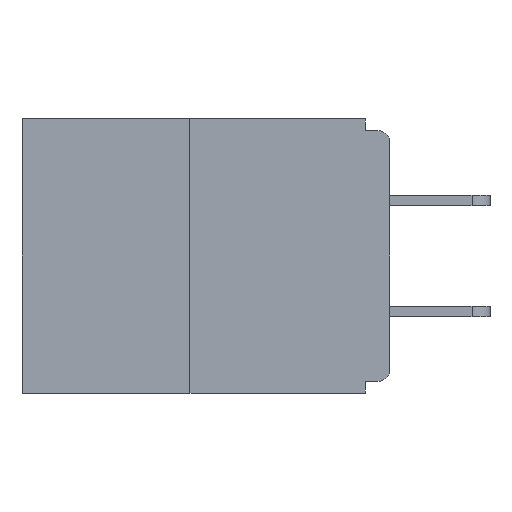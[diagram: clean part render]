
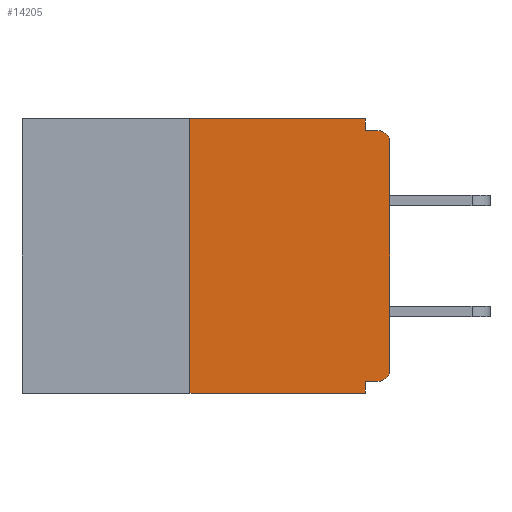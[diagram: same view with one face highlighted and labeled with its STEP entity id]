
A CAD part, left-side view. The second image highlights one B-rep face of the part: STEP entity #14205.
In plain terms, the highlighted planar face has unit normal (-1, 0, 0).
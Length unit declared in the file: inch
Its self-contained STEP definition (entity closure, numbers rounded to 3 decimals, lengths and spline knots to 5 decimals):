
#158 = CARTESIAN_POINT ( 'NONE',  ( 0., 0.015, -0.328 ) ) ;
#215 = CARTESIAN_POINT ( 'NONE',  ( 0., 0.25, 0. ) ) ;
#229 = EDGE_CURVE ( 'NONE', #11083, #8992, #6407, .T. ) ;
#235 = CARTESIAN_POINT ( 'NONE',  ( 0., 0.46, 0. ) ) ;
#699 = VECTOR ( 'NONE', #16931, 39.37008 ) ;
#839 = AXIS2_PLACEMENT_3D ( 'NONE', #7268, #9706, #13663 ) ;
#892 = VECTOR ( 'NONE', #11064, 39.37008 ) ;
#1254 = AXIS2_PLACEMENT_3D ( 'NONE', #10747, #15986, #8151 ) ;
#1256 = EDGE_CURVE ( 'NONE', #16691, #2936, #14068, .T. ) ;
#1741 = LINE ( 'NONE', #15733, #16290 ) ;
#1963 = DIRECTION ( 'NONE',  ( 0., -1., 0. ) ) ;
#2373 = AXIS2_PLACEMENT_3D ( 'NONE', #235, #15900, #2835 ) ;
#2428 = ORIENTED_EDGE ( 'NONE', *, *, #229, .F. ) ;
#2693 = LINE ( 'NONE', #5955, #9291 ) ;
#2835 = DIRECTION ( 'NONE',  ( 0., 0., -1. ) ) ;
#2936 = VERTEX_POINT ( 'NONE', #3466 ) ;
#3057 = EDGE_CURVE ( 'NONE', #14549, #4964, #15224, .T. ) ;
#3086 = LINE ( 'NONE', #5549, #16845 ) ;
#3451 = CARTESIAN_POINT ( 'NONE',  ( 0., 0.25, 0. ) ) ;
#3466 = CARTESIAN_POINT ( 'NONE',  ( 0., 0., -0.03 ) ) ;
#3746 = EDGE_CURVE ( 'NONE', #7110, #16691, #11566, .T. ) ;
#3866 = DIRECTION ( 'NONE',  ( 0., 0., -1. ) ) ;
#4085 = CARTESIAN_POINT ( 'NONE',  ( 0., 0.25, -0.343 ) ) ;
#4459 = CARTESIAN_POINT ( 'NONE',  ( 0., 0.031, -0.328 ) ) ;
#4520 = VECTOR ( 'NONE', #1963, 39.37008 ) ;
#4844 = EDGE_CURVE ( 'NONE', #7110, #6276, #3086, .T. ) ;
#4888 = DIRECTION ( 'NONE',  ( 0., -1., 0. ) ) ;
#4964 = VERTEX_POINT ( 'NONE', #3451 ) ;
#5214 = DIRECTION ( 'NONE',  ( 0., 0., 1. ) ) ;
#5549 = CARTESIAN_POINT ( 'NONE',  ( 0., 0., -0.328 ) ) ;
#5955 = CARTESIAN_POINT ( 'NONE',  ( 0., 0.46, 0. ) ) ;
#6276 = VERTEX_POINT ( 'NONE', #4459 ) ;
#6407 = LINE ( 'NONE', #13141, #699 ) ;
#6719 = PLANE ( 'NONE',  #2373 ) ;
#6796 = ORIENTED_EDGE ( 'NONE', *, *, #3746, .T. ) ;
#6981 = CARTESIAN_POINT ( 'NONE',  ( 0., 0., -0.313 ) ) ;
#7110 = VERTEX_POINT ( 'NONE', #158 ) ;
#7268 = CARTESIAN_POINT ( 'NONE',  ( 0., 0.015, -0.03 ) ) ;
#7637 = CIRCLE ( 'NONE', #839, 0.015 ) ;
#8071 = CARTESIAN_POINT ( 'NONE',  ( 0., 0.031, -0.343 ) ) ;
#8128 = EDGE_CURVE ( 'NONE', #8992, #9501, #16597, .T. ) ;
#8151 = DIRECTION ( 'NONE',  ( 0., 0., -1. ) ) ;
#8404 = EDGE_LOOP ( 'NONE', ( #16048, #16603, #12845, #13009, #9091, #6796, #16821, #12094, #10061, #2428 ) ) ;
#8992 = VERTEX_POINT ( 'NONE', #13376 ) ;
#9091 = ORIENTED_EDGE ( 'NONE', *, *, #4844, .F. ) ;
#9167 = VECTOR ( 'NONE', #5214, 39.37008 ) ;
#9291 = VECTOR ( 'NONE', #4888, 39.37008 ) ;
#9501 = VERTEX_POINT ( 'NONE', #10164 ) ;
#9706 = DIRECTION ( 'NONE',  ( -1., 0., 0. ) ) ;
#10061 = ORIENTED_EDGE ( 'NONE', *, *, #8128, .F. ) ;
#10164 = CARTESIAN_POINT ( 'NONE',  ( 0., 0.015, -0.015 ) ) ;
#10503 = DIRECTION ( 'NONE',  ( 0., -1., 0. ) ) ;
#10747 = CARTESIAN_POINT ( 'NONE',  ( 0., 0.015, -0.313 ) ) ;
#10772 = CARTESIAN_POINT ( 'NONE',  ( 0., 0.46, -0.343 ) ) ;
#11058 = DIRECTION ( 'NONE',  ( 0., 1., 0. ) ) ;
#11064 = DIRECTION ( 'NONE',  ( 0., 0., 1. ) ) ;
#11075 = VERTEX_POINT ( 'NONE', #8071 ) ;
#11083 = VERTEX_POINT ( 'NONE', #14409 ) ;
#11508 = VECTOR ( 'NONE', #10503, 39.37008 ) ;
#11547 = EDGE_CURVE ( 'NONE', #6276, #11075, #1741, .T. ) ;
#11566 = CIRCLE ( 'NONE', #1254, 0.015 ) ;
#11839 = CARTESIAN_POINT ( 'NONE',  ( 0., 0., -0.015 ) ) ;
#12094 = ORIENTED_EDGE ( 'NONE', *, *, #12555, .T. ) ;
#12244 = EDGE_CURVE ( 'NONE', #4964, #11083, #2693, .T. ) ;
#12555 = EDGE_CURVE ( 'NONE', #2936, #9501, #7637, .T. ) ;
#12845 = ORIENTED_EDGE ( 'NONE', *, *, #16452, .T. ) ;
#13009 = ORIENTED_EDGE ( 'NONE', *, *, #11547, .F. ) ;
#13141 = CARTESIAN_POINT ( 'NONE',  ( 0., 0.031, 0. ) ) ;
#13342 = LINE ( 'NONE', #10772, #4520 ) ;
#13376 = CARTESIAN_POINT ( 'NONE',  ( 0., 0.031, -0.015 ) ) ;
#13412 = FACE_OUTER_BOUND ( 'NONE', #8404, .T. ) ;
#13663 = DIRECTION ( 'NONE',  ( 0., 0., -1. ) ) ;
#14068 = LINE ( 'NONE', #14439, #9167 ) ;
#14205 = ADVANCED_FACE ( 'NONE', ( #13412 ), #6719, .F. ) ;
#14409 = CARTESIAN_POINT ( 'NONE',  ( 0., 0.031, 0. ) ) ;
#14439 = CARTESIAN_POINT ( 'NONE',  ( 0., 0., 0. ) ) ;
#14549 = VERTEX_POINT ( 'NONE', #4085 ) ;
#15224 = LINE ( 'NONE', #215, #892 ) ;
#15733 = CARTESIAN_POINT ( 'NONE',  ( 0., 0.031, -0.343 ) ) ;
#15900 = DIRECTION ( 'NONE',  ( 1., 0., 0. ) ) ;
#15986 = DIRECTION ( 'NONE',  ( -1., 0., 0. ) ) ;
#16048 = ORIENTED_EDGE ( 'NONE', *, *, #12244, .F. ) ;
#16290 = VECTOR ( 'NONE', #3866, 39.37008 ) ;
#16452 = EDGE_CURVE ( 'NONE', #14549, #11075, #13342, .T. ) ;
#16597 = LINE ( 'NONE', #11839, #11508 ) ;
#16603 = ORIENTED_EDGE ( 'NONE', *, *, #3057, .F. ) ;
#16691 = VERTEX_POINT ( 'NONE', #6981 ) ;
#16821 = ORIENTED_EDGE ( 'NONE', *, *, #1256, .T. ) ;
#16845 = VECTOR ( 'NONE', #11058, 39.37008 ) ;
#16931 = DIRECTION ( 'NONE',  ( 0., 0., -1. ) ) ;
